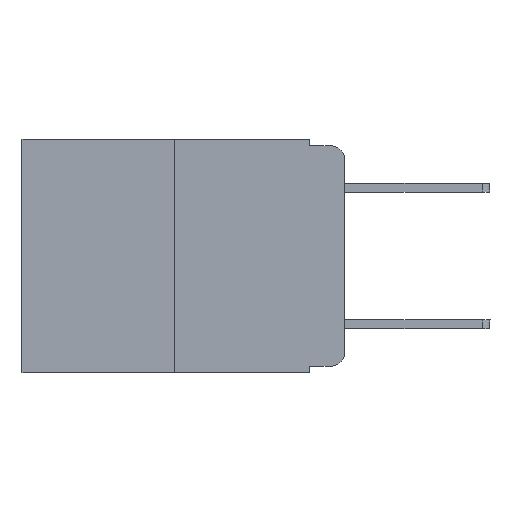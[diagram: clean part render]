
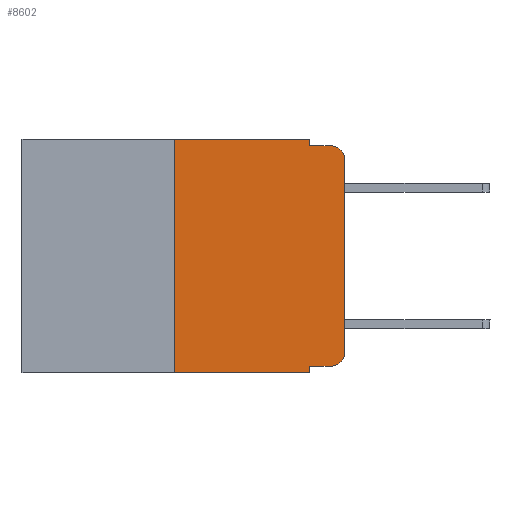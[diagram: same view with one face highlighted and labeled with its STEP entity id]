
A CAD part, left-side view. The second image highlights one B-rep face of the part: STEP entity #8602.
In plain terms, the highlighted planar face has unit normal (-1, 0, 0).
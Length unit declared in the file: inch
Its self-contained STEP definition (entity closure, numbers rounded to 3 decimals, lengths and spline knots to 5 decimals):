
#88 = ORIENTED_EDGE ( 'NONE', *, *, #8796, .T. ) ;
#380 = CARTESIAN_POINT ( 'NONE',  ( 0., 0.25, -0.343 ) ) ;
#1003 = DIRECTION ( 'NONE',  ( 0., 0., -1. ) ) ;
#1100 = CARTESIAN_POINT ( 'NONE',  ( 0., 0.473, 0. ) ) ;
#1199 = DIRECTION ( 'NONE',  ( 1., 0., 0. ) ) ;
#1237 = LINE ( 'NONE', #16130, #4247 ) ;
#1480 = DIRECTION ( 'NONE',  ( 0., 0., -1. ) ) ;
#1507 = CARTESIAN_POINT ( 'NONE',  ( 0., 0., -0.03 ) ) ;
#1538 = DIRECTION ( 'NONE',  ( 0., -1., 0. ) ) ;
#1577 = ORIENTED_EDGE ( 'NONE', *, *, #16055, .F. ) ;
#1795 = VECTOR ( 'NONE', #3419, 39.37008 ) ;
#1922 = CARTESIAN_POINT ( 'NONE',  ( 0., 0.051, 0. ) ) ;
#2046 = CARTESIAN_POINT ( 'NONE',  ( 0., 0.25, 0. ) ) ;
#2097 = VECTOR ( 'NONE', #3780, 39.37008 ) ;
#2142 = CARTESIAN_POINT ( 'NONE',  ( 0., 0.02, -0.01 ) ) ;
#2168 = CARTESIAN_POINT ( 'NONE',  ( 0., 0.051, -0.01 ) ) ;
#2484 = PLANE ( 'NONE',  #13876 ) ;
#2493 = ORIENTED_EDGE ( 'NONE', *, *, #18797, .T. ) ;
#2526 = DIRECTION ( 'NONE',  ( 0., 0., 1. ) ) ;
#2593 = EDGE_CURVE ( 'NONE', #7319, #12133, #1237, .T. ) ;
#2902 = ORIENTED_EDGE ( 'NONE', *, *, #10922, .F. ) ;
#3171 = ORIENTED_EDGE ( 'NONE', *, *, #2593, .T. ) ;
#3314 = VERTEX_POINT ( 'NONE', #2168 ) ;
#3376 = ORIENTED_EDGE ( 'NONE', *, *, #12779, .F. ) ;
#3419 = DIRECTION ( 'NONE',  ( 0., -1., 0. ) ) ;
#3780 = DIRECTION ( 'NONE',  ( 0., 0., -1. ) ) ;
#3986 = ORIENTED_EDGE ( 'NONE', *, *, #6963, .F. ) ;
#4161 = EDGE_LOOP ( 'NONE', ( #3171, #88, #2902, #3376, #1577, #9484, #2493, #3986, #8806, #9776 ) ) ;
#4247 = VECTOR ( 'NONE', #2526, 39.37008 ) ;
#4883 = VERTEX_POINT ( 'NONE', #5497 ) ;
#5393 = CARTESIAN_POINT ( 'NONE',  ( 0., 0.051, -0.343 ) ) ;
#5497 = CARTESIAN_POINT ( 'NONE',  ( 0., 0.051, 0. ) ) ;
#6398 = EDGE_CURVE ( 'NONE', #17538, #12392, #16840, .T. ) ;
#6475 = VERTEX_POINT ( 'NONE', #2142 ) ;
#6500 = CARTESIAN_POINT ( 'NONE',  ( 0., 0.02, -0.333 ) ) ;
#6963 = EDGE_CURVE ( 'NONE', #17538, #12896, #18681, .T. ) ;
#6970 = CARTESIAN_POINT ( 'NONE',  ( 0., 0.25, 0. ) ) ;
#7303 = AXIS2_PLACEMENT_3D ( 'NONE', #9032, #19324, #1480 ) ;
#7319 = VERTEX_POINT ( 'NONE', #10612 ) ;
#7461 = CARTESIAN_POINT ( 'NONE',  ( 0., 0.051, 0. ) ) ;
#7507 = VERTEX_POINT ( 'NONE', #6970 ) ;
#7575 = DIRECTION ( 'NONE',  ( 0., -1., 0. ) ) ;
#7717 = CARTESIAN_POINT ( 'NONE',  ( 0., 0.051, -0.333 ) ) ;
#8602 = ADVANCED_FACE ( 'NONE', ( #14435 ), #2484, .F. ) ;
#8685 = VECTOR ( 'NONE', #15013, 39.37008 ) ;
#8796 = EDGE_CURVE ( 'NONE', #12133, #6475, #8872, .T. ) ;
#8806 = ORIENTED_EDGE ( 'NONE', *, *, #6398, .T. ) ;
#8872 = CIRCLE ( 'NONE', #7303, 0.02 ) ;
#9014 = DIRECTION ( 'NONE',  ( -1., 0., 0. ) ) ;
#9032 = CARTESIAN_POINT ( 'NONE',  ( 0., 0.02, -0.03 ) ) ;
#9062 = CARTESIAN_POINT ( 'NONE',  ( 0., 0.051, -0.333 ) ) ;
#9183 = LINE ( 'NONE', #19282, #17283 ) ;
#9484 = ORIENTED_EDGE ( 'NONE', *, *, #15336, .F. ) ;
#9591 = LINE ( 'NONE', #2046, #11538 ) ;
#9776 = ORIENTED_EDGE ( 'NONE', *, *, #17891, .T. ) ;
#10017 = VERTEX_POINT ( 'NONE', #380 ) ;
#10612 = CARTESIAN_POINT ( 'NONE',  ( 0., 0., -0.313 ) ) ;
#10865 = DIRECTION ( 'NONE',  ( 0., 0., 1. ) ) ;
#10922 = EDGE_CURVE ( 'NONE', #3314, #6475, #12383, .T. ) ;
#11538 = VECTOR ( 'NONE', #10865, 39.37008 ) ;
#12133 = VERTEX_POINT ( 'NONE', #1507 ) ;
#12343 = DIRECTION ( 'NONE',  ( 0., 0., -1. ) ) ;
#12383 = LINE ( 'NONE', #13651, #15512 ) ;
#12392 = VERTEX_POINT ( 'NONE', #6500 ) ;
#12779 = EDGE_CURVE ( 'NONE', #4883, #3314, #14911, .T. ) ;
#12896 = VERTEX_POINT ( 'NONE', #5393 ) ;
#13651 = CARTESIAN_POINT ( 'NONE',  ( 0., 0.051, -0.01 ) ) ;
#13808 = AXIS2_PLACEMENT_3D ( 'NONE', #16750, #9014, #12343 ) ;
#13876 = AXIS2_PLACEMENT_3D ( 'NONE', #17571, #1199, #1003 ) ;
#14129 = CIRCLE ( 'NONE', #13808, 0.02 ) ;
#14435 = FACE_OUTER_BOUND ( 'NONE', #4161, .T. ) ;
#14911 = LINE ( 'NONE', #7461, #8685 ) ;
#15013 = DIRECTION ( 'NONE',  ( 0., 0., -1. ) ) ;
#15336 = EDGE_CURVE ( 'NONE', #10017, #7507, #9591, .T. ) ;
#15512 = VECTOR ( 'NONE', #7575, 39.37008 ) ;
#16055 = EDGE_CURVE ( 'NONE', #7507, #4883, #16196, .T. ) ;
#16130 = CARTESIAN_POINT ( 'NONE',  ( 0., 0., 0. ) ) ;
#16196 = LINE ( 'NONE', #1100, #16261 ) ;
#16261 = VECTOR ( 'NONE', #17670, 39.37008 ) ;
#16750 = CARTESIAN_POINT ( 'NONE',  ( 0., 0.02, -0.313 ) ) ;
#16840 = LINE ( 'NONE', #7717, #1795 ) ;
#17283 = VECTOR ( 'NONE', #1538, 39.37008 ) ;
#17538 = VERTEX_POINT ( 'NONE', #9062 ) ;
#17571 = CARTESIAN_POINT ( 'NONE',  ( 0., 0.473, 0. ) ) ;
#17670 = DIRECTION ( 'NONE',  ( 0., -1., 0. ) ) ;
#17891 = EDGE_CURVE ( 'NONE', #12392, #7319, #14129, .T. ) ;
#18681 = LINE ( 'NONE', #1922, #2097 ) ;
#18797 = EDGE_CURVE ( 'NONE', #10017, #12896, #9183, .T. ) ;
#19282 = CARTESIAN_POINT ( 'NONE',  ( 0., 0.473, -0.343 ) ) ;
#19324 = DIRECTION ( 'NONE',  ( -1., 0., 0. ) ) ;
